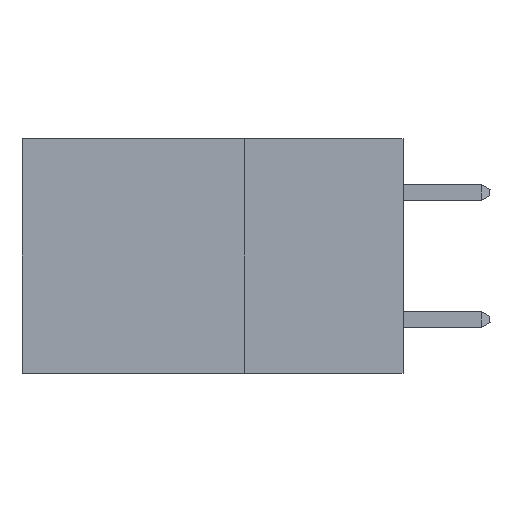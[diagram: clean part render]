
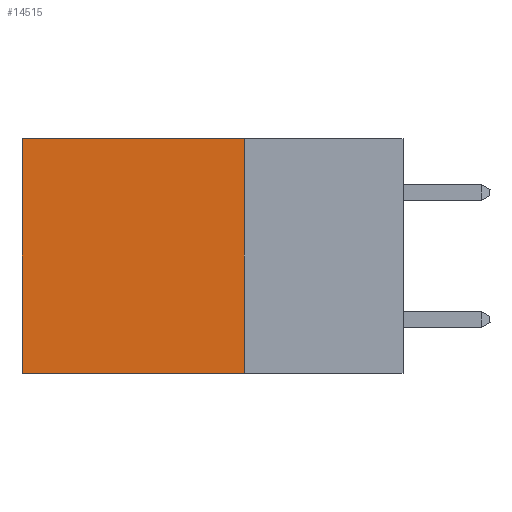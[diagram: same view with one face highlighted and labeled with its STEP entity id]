
A CAD part, left-side view. The second image highlights one B-rep face of the part: STEP entity #14515.
In plain terms, the highlighted planar face has unit normal (-1, 0, 0).
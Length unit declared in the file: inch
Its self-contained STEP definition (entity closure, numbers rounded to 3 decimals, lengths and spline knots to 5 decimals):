
#2186 = VERTEX_POINT ( 'NONE', #8813 ) ;
#2745 = ORIENTED_EDGE ( 'NONE', *, *, #16270, .F. ) ;
#3003 = VERTEX_POINT ( 'NONE', #24887 ) ;
#3504 = AXIS2_PLACEMENT_3D ( 'NONE', #9094, #19359, #24696 ) ;
#3748 = ORIENTED_EDGE ( 'NONE', *, *, #6460, .F. ) ;
#6430 = DIRECTION ( 'NONE',  ( 0., 0., -1. ) ) ;
#6460 = EDGE_CURVE ( 'NONE', #15013, #2186, #30279, .T. ) ;
#8813 = CARTESIAN_POINT ( 'NONE',  ( 0.2875, 0.25, -0.37 ) ) ;
#9094 = CARTESIAN_POINT ( 'NONE',  ( 0.2875, 0.25, 0. ) ) ;
#12329 = CARTESIAN_POINT ( 'NONE',  ( 0.2875, 0.25, 0. ) ) ;
#12656 = CARTESIAN_POINT ( 'NONE',  ( 0.2875, 0.25, 0. ) ) ;
#13207 = VECTOR ( 'NONE', #6430, 39.37008 ) ;
#14515 = ADVANCED_FACE ( 'NONE', ( #21248 ), #22447, .F. ) ;
#15013 = VERTEX_POINT ( 'NONE', #12329 ) ;
#15370 = ORIENTED_EDGE ( 'NONE', *, *, #30879, .T. ) ;
#16270 = EDGE_CURVE ( 'NONE', #2186, #3003, #35852, .T. ) ;
#18211 = CARTESIAN_POINT ( 'NONE',  ( 0.2875, 0.6, 0. ) ) ;
#19217 = VECTOR ( 'NONE', #33122, 39.37008 ) ;
#19359 = DIRECTION ( 'NONE',  ( 1., 0., 0. ) ) ;
#21248 = FACE_OUTER_BOUND ( 'NONE', #30040, .T. ) ;
#22447 = PLANE ( 'NONE',  #3504 ) ;
#23400 = LINE ( 'NONE', #12656, #19217 ) ;
#24171 = CARTESIAN_POINT ( 'NONE',  ( 0.2875, 0.25, -0.37 ) ) ;
#24696 = DIRECTION ( 'NONE',  ( 0., 0., -1. ) ) ;
#24887 = CARTESIAN_POINT ( 'NONE',  ( 0.2875, 0.6, -0.37 ) ) ;
#26653 = CARTESIAN_POINT ( 'NONE',  ( 0.2875, 0.25, 0. ) ) ;
#28078 = LINE ( 'NONE', #18211, #34980 ) ;
#28618 = EDGE_CURVE ( 'NONE', #15013, #29811, #23400, .T. ) ;
#29811 = VERTEX_POINT ( 'NONE', #35417 ) ;
#30040 = EDGE_LOOP ( 'NONE', ( #15370, #2745, #3748, #33046 ) ) ;
#30279 = LINE ( 'NONE', #26653, #13207 ) ;
#30879 = EDGE_CURVE ( 'NONE', #29811, #3003, #28078, .T. ) ;
#31728 = VECTOR ( 'NONE', #33034, 39.37008 ) ;
#33034 = DIRECTION ( 'NONE',  ( 0., 1., 0. ) ) ;
#33046 = ORIENTED_EDGE ( 'NONE', *, *, #28618, .T. ) ;
#33122 = DIRECTION ( 'NONE',  ( 0., 1., 0. ) ) ;
#34980 = VECTOR ( 'NONE', #35423, 39.37008 ) ;
#35417 = CARTESIAN_POINT ( 'NONE',  ( 0.2875, 0.6, 0. ) ) ;
#35423 = DIRECTION ( 'NONE',  ( 0., 0., -1. ) ) ;
#35852 = LINE ( 'NONE', #24171, #31728 ) ;
